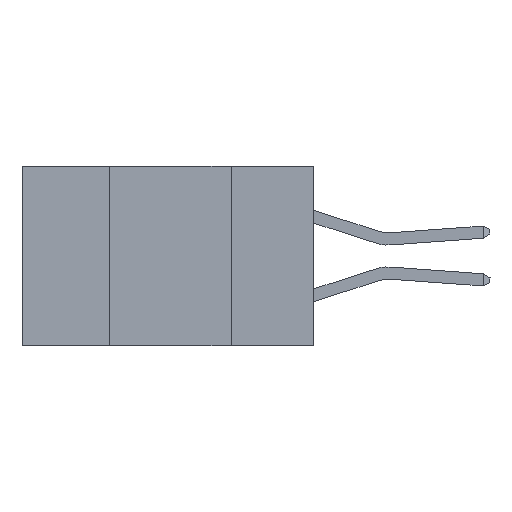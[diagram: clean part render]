
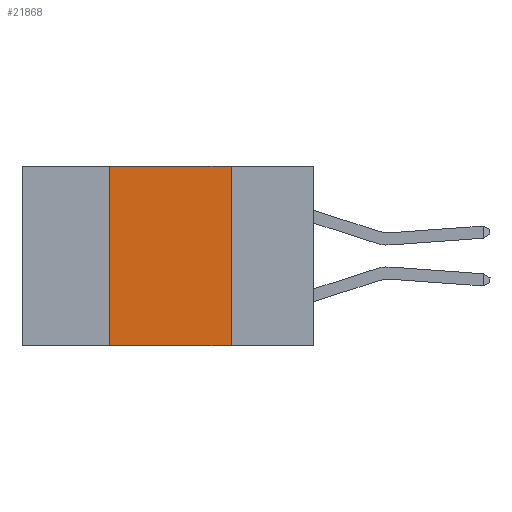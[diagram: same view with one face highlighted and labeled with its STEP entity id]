
A CAD part, left-side view. The second image highlights one B-rep face of the part: STEP entity #21868.
In plain terms, the highlighted planar face has unit normal (-1, 0, 0).
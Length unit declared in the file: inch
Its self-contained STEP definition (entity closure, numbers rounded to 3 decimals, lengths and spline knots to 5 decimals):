
#1375 = EDGE_CURVE ( 'NONE', #12751, #37019, #15111, .T. ) ;
#2392 = LINE ( 'NONE', #19399, #23101 ) ;
#3226 = PLANE ( 'NONE',  #16274 ) ;
#4261 = DIRECTION ( 'NONE',  ( 0., 0., -1. ) ) ;
#5150 = EDGE_CURVE ( 'NONE', #12751, #32292, #2392, .T. ) ;
#6243 = CARTESIAN_POINT ( 'NONE',  ( 0., 0.17, 0. ) ) ;
#6678 = VECTOR ( 'NONE', #25687, 39.37008 ) ;
#7024 = CARTESIAN_POINT ( 'NONE',  ( 0., 0.6, 0. ) ) ;
#7833 = VERTEX_POINT ( 'NONE', #6243 ) ;
#8295 = LINE ( 'NONE', #8511, #33804 ) ;
#8511 = CARTESIAN_POINT ( 'NONE',  ( 0., 0.17, 0. ) ) ;
#8699 = ORIENTED_EDGE ( 'NONE', *, *, #5150, .F. ) ;
#9807 = CARTESIAN_POINT ( 'NONE',  ( 0., 0.6, 0. ) ) ;
#10577 = CARTESIAN_POINT ( 'NONE',  ( 0., 0.6, -0.37 ) ) ;
#11406 = DIRECTION ( 'NONE',  ( 0., 0., -1. ) ) ;
#12286 = EDGE_CURVE ( 'NONE', #7833, #37019, #8295, .T. ) ;
#12751 = VERTEX_POINT ( 'NONE', #34187 ) ;
#13709 = EDGE_LOOP ( 'NONE', ( #32487, #18672, #8699, #13984 ) ) ;
#13984 = ORIENTED_EDGE ( 'NONE', *, *, #1375, .T. ) ;
#15111 = LINE ( 'NONE', #10577, #21899 ) ;
#15712 = DIRECTION ( 'NONE',  ( 1., 0., 0. ) ) ;
#16274 = AXIS2_PLACEMENT_3D ( 'NONE', #9807, #15712, #4261 ) ;
#16360 = EDGE_CURVE ( 'NONE', #32292, #7833, #20201, .T. ) ;
#18672 = ORIENTED_EDGE ( 'NONE', *, *, #16360, .F. ) ;
#19399 = CARTESIAN_POINT ( 'NONE',  ( 0., 0.42, 0. ) ) ;
#20201 = LINE ( 'NONE', #7024, #6678 ) ;
#21868 = ADVANCED_FACE ( 'NONE', ( #30736 ), #3226, .F. ) ;
#21899 = VECTOR ( 'NONE', #30548, 39.37008 ) ;
#23101 = VECTOR ( 'NONE', #25246, 39.37008 ) ;
#25246 = DIRECTION ( 'NONE',  ( 0., 0., 1. ) ) ;
#25687 = DIRECTION ( 'NONE',  ( 0., -1., 0. ) ) ;
#30548 = DIRECTION ( 'NONE',  ( 0., -1., 0. ) ) ;
#30736 = FACE_OUTER_BOUND ( 'NONE', #13709, .T. ) ;
#32214 = CARTESIAN_POINT ( 'NONE',  ( 0., 0.42, 0. ) ) ;
#32292 = VERTEX_POINT ( 'NONE', #32214 ) ;
#32487 = ORIENTED_EDGE ( 'NONE', *, *, #12286, .F. ) ;
#33804 = VECTOR ( 'NONE', #11406, 39.37008 ) ;
#33992 = CARTESIAN_POINT ( 'NONE',  ( 0., 0.17, -0.37 ) ) ;
#34187 = CARTESIAN_POINT ( 'NONE',  ( 0., 0.42, -0.37 ) ) ;
#37019 = VERTEX_POINT ( 'NONE', #33992 ) ;
